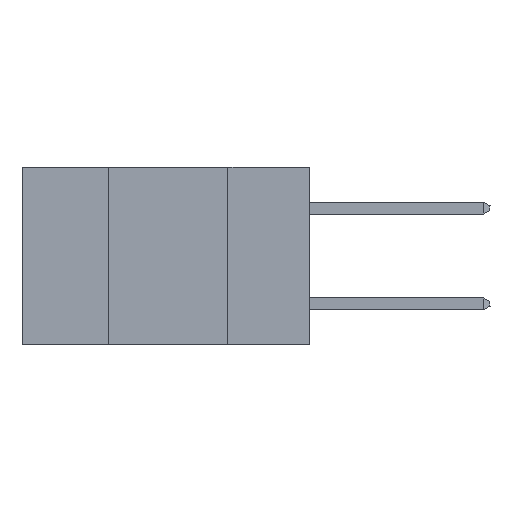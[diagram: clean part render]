
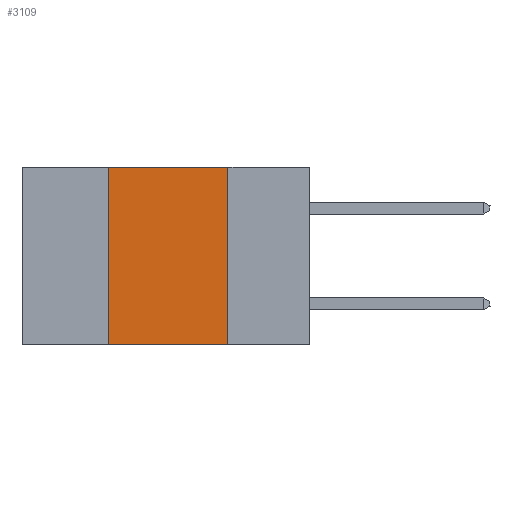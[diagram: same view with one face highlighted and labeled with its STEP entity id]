
A CAD part, left-side view. The second image highlights one B-rep face of the part: STEP entity #3109.
In plain terms, the highlighted planar face has unit normal (-1, 0, 0).
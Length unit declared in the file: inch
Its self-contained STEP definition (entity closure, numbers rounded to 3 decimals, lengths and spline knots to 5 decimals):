
#636 = DIRECTION ( 'NONE',  ( 1., 0., 0. ) ) ;
#686 = DIRECTION ( 'NONE',  ( 0., -1., 0. ) ) ;
#1600 = CARTESIAN_POINT ( 'NONE',  ( 0., 0.17, 0. ) ) ;
#3109 = ADVANCED_FACE ( 'NONE', ( #13636 ), #12372, .F. ) ;
#5218 = CARTESIAN_POINT ( 'NONE',  ( 0., 0.17, -0.37 ) ) ;
#5516 = VECTOR ( 'NONE', #20441, 39.37008 ) ;
#5559 = DIRECTION ( 'NONE',  ( 0., 0., -1. ) ) ;
#5937 = CARTESIAN_POINT ( 'NONE',  ( 0., 0.42, 0. ) ) ;
#6518 = ORIENTED_EDGE ( 'NONE', *, *, #10672, .T. ) ;
#6540 = CARTESIAN_POINT ( 'NONE',  ( 0., 0.6, 0. ) ) ;
#6877 = LINE ( 'NONE', #1600, #16636 ) ;
#7237 = EDGE_CURVE ( 'NONE', #9025, #20043, #6877, .T. ) ;
#8814 = CARTESIAN_POINT ( 'NONE',  ( 0., 0.6, -0.37 ) ) ;
#9025 = VERTEX_POINT ( 'NONE', #17054 ) ;
#9166 = VERTEX_POINT ( 'NONE', #20076 ) ;
#9562 = VERTEX_POINT ( 'NONE', #22999 ) ;
#10672 = EDGE_CURVE ( 'NONE', #9166, #20043, #15863, .T. ) ;
#10702 = ORIENTED_EDGE ( 'NONE', *, *, #14602, .F. ) ;
#11062 = LINE ( 'NONE', #6540, #20753 ) ;
#12372 = PLANE ( 'NONE',  #12828 ) ;
#12828 = AXIS2_PLACEMENT_3D ( 'NONE', #21992, #636, #14333 ) ;
#13619 = EDGE_LOOP ( 'NONE', ( #14707, #19681, #10702, #6518 ) ) ;
#13636 = FACE_OUTER_BOUND ( 'NONE', #13619, .T. ) ;
#14260 = VECTOR ( 'NONE', #19634, 39.37008 ) ;
#14333 = DIRECTION ( 'NONE',  ( 0., 0., -1. ) ) ;
#14602 = EDGE_CURVE ( 'NONE', #9166, #9562, #24509, .T. ) ;
#14707 = ORIENTED_EDGE ( 'NONE', *, *, #7237, .F. ) ;
#15863 = LINE ( 'NONE', #8814, #5516 ) ;
#16636 = VECTOR ( 'NONE', #5559, 39.37008 ) ;
#17054 = CARTESIAN_POINT ( 'NONE',  ( 0., 0.17, 0. ) ) ;
#19634 = DIRECTION ( 'NONE',  ( 0., 0., 1. ) ) ;
#19681 = ORIENTED_EDGE ( 'NONE', *, *, #22942, .F. ) ;
#20043 = VERTEX_POINT ( 'NONE', #5218 ) ;
#20076 = CARTESIAN_POINT ( 'NONE',  ( 0., 0.42, -0.37 ) ) ;
#20441 = DIRECTION ( 'NONE',  ( 0., -1., 0. ) ) ;
#20753 = VECTOR ( 'NONE', #686, 39.37008 ) ;
#21992 = CARTESIAN_POINT ( 'NONE',  ( 0., 0.6, 0. ) ) ;
#22942 = EDGE_CURVE ( 'NONE', #9562, #9025, #11062, .T. ) ;
#22999 = CARTESIAN_POINT ( 'NONE',  ( 0., 0.42, 0. ) ) ;
#24509 = LINE ( 'NONE', #5937, #14260 ) ;
